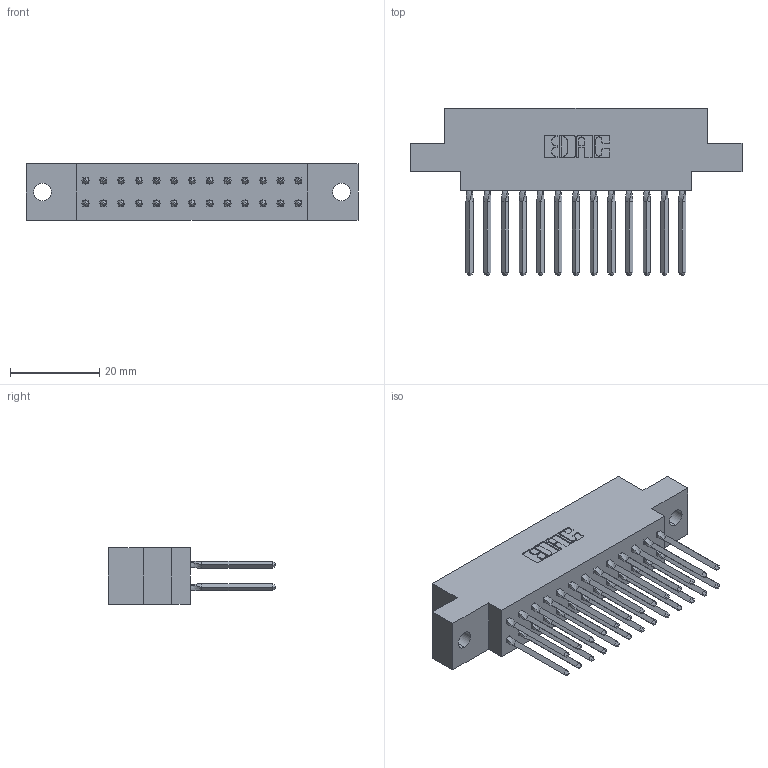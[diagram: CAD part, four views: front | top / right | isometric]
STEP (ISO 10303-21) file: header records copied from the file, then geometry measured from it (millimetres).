
FILE_DESCRIPTION (( 'STEP AP203' ), '1' );
FILE_NAME ('317-026-540-804.STEP', '2020-02-27T18:49:51', ( '' ), ( '' ), 'SwSTEP 2.0', 'SolidWorks 2016', '' );
FILE_SCHEMA (( 'CONFIG_CONTROL_DESIGN' ));
Length unit declared in the file: inch
Products named in the file (3): 317-026-540-804; 317 Part_.156 Dia - TH; 317-290-001_540
Assembly tree (27 placements, depth 2):
  317-026-540-804
    317 Part_.156 Dia - TH
    317-290-001_540  x26
Bounding box: 74.22 x 37.34 x 12.7 mm (x, y, z)
Volume: 11387.8 mm3; surface area: 15707.8 mm2
Topology: 27 solids, 27 shells, 2416 faces, 6697 edges, 4316 vertices
Faces by surface type: plane 1956, cylinder 356, bspline 104
Entity records: 22840 total; most frequent: CARTESIAN_POINT 4395, ORIENTED_EDGE 3894, DIRECTION 3253, EDGE_CURVE 1947, LINE 1691, VECTOR 1691, VERTEX_POINT 1291, AXIS2_PLACEMENT_3D 781
